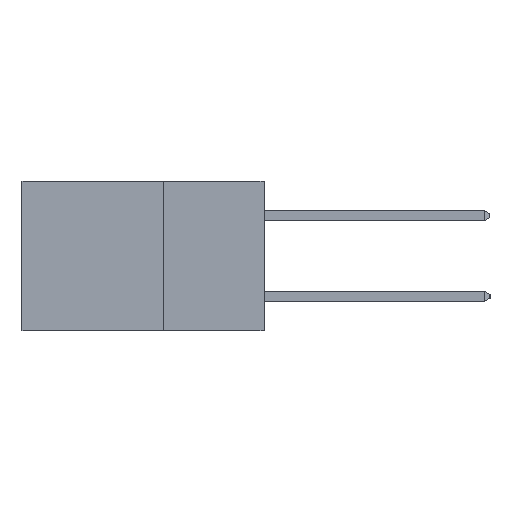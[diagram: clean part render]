
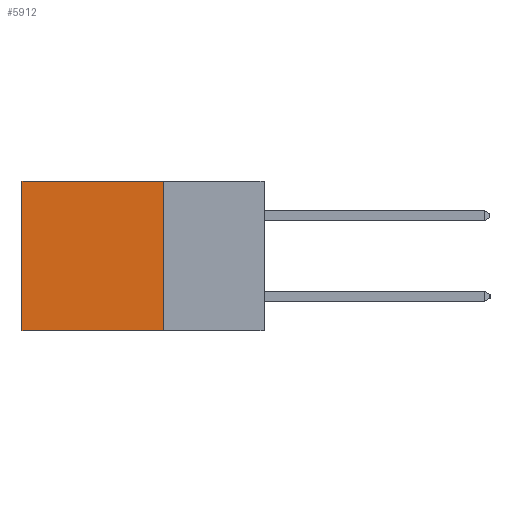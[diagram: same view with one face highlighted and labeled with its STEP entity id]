
A CAD part, left-side view. The second image highlights one B-rep face of the part: STEP entity #5912.
In plain terms, the highlighted planar face has unit normal (-1, 0, 0).
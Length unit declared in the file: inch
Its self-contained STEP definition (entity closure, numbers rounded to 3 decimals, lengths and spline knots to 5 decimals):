
#74 = DIRECTION ( 'NONE',  ( 0., 0., -1. ) ) ;
#512 = CARTESIAN_POINT ( 'NONE',  ( 0.2615, 0.25, -0.37 ) ) ;
#1119 = LINE ( 'NONE', #2760, #7831 ) ;
#1489 = CARTESIAN_POINT ( 'NONE',  ( 0.2615, 0.25, 0. ) ) ;
#1508 = DIRECTION ( 'NONE',  ( 0., 0., -1. ) ) ;
#1572 = LINE ( 'NONE', #512, #10330 ) ;
#2566 = PLANE ( 'NONE',  #3151 ) ;
#2760 = CARTESIAN_POINT ( 'NONE',  ( 0.2615, 0.25, -0.37 ) ) ;
#3151 = AXIS2_PLACEMENT_3D ( 'NONE', #3512, #10119, #5229 ) ;
#3495 = CARTESIAN_POINT ( 'NONE',  ( 0.2615, 0.25, -0.37 ) ) ;
#3512 = CARTESIAN_POINT ( 'NONE',  ( 0.2615, 0.25, -0.37 ) ) ;
#4608 = EDGE_LOOP ( 'NONE', ( #7657, #6684, #6262, #6274 ) ) ;
#4734 = VERTEX_POINT ( 'NONE', #8314 ) ;
#4958 = LINE ( 'NONE', #10411, #9104 ) ;
#4966 = FACE_OUTER_BOUND ( 'NONE', #4608, .T. ) ;
#5229 = DIRECTION ( 'NONE',  ( 0., 0., -1. ) ) ;
#5588 = CARTESIAN_POINT ( 'NONE',  ( 0.2615, 0.6, -0.37 ) ) ;
#5912 = ADVANCED_FACE ( 'NONE', ( #4966 ), #2566, .F. ) ;
#5965 = VERTEX_POINT ( 'NONE', #6165 ) ;
#6045 = EDGE_CURVE ( 'NONE', #6801, #4734, #1119, .T. ) ;
#6165 = CARTESIAN_POINT ( 'NONE',  ( 0.2615, 0.6, 0. ) ) ;
#6214 = EDGE_CURVE ( 'NONE', #5965, #4734, #11045, .T. ) ;
#6262 = ORIENTED_EDGE ( 'NONE', *, *, #7633, .F. ) ;
#6274 = ORIENTED_EDGE ( 'NONE', *, *, #7068, .T. ) ;
#6684 = ORIENTED_EDGE ( 'NONE', *, *, #6045, .F. ) ;
#6801 = VERTEX_POINT ( 'NONE', #3495 ) ;
#7068 = EDGE_CURVE ( 'NONE', #11093, #5965, #4958, .T. ) ;
#7633 = EDGE_CURVE ( 'NONE', #11093, #6801, #1572, .T. ) ;
#7657 = ORIENTED_EDGE ( 'NONE', *, *, #6214, .T. ) ;
#7831 = VECTOR ( 'NONE', #7862, 39.37008 ) ;
#7862 = DIRECTION ( 'NONE',  ( 0., 1., 0. ) ) ;
#8314 = CARTESIAN_POINT ( 'NONE',  ( 0.2615, 0.6, -0.37 ) ) ;
#8712 = VECTOR ( 'NONE', #74, 39.37008 ) ;
#8860 = DIRECTION ( 'NONE',  ( 0., 1., 0. ) ) ;
#9104 = VECTOR ( 'NONE', #8860, 39.37008 ) ;
#10119 = DIRECTION ( 'NONE',  ( 1., 0., 0. ) ) ;
#10330 = VECTOR ( 'NONE', #1508, 39.37008 ) ;
#10411 = CARTESIAN_POINT ( 'NONE',  ( 0.2615, 0.25, 0. ) ) ;
#11045 = LINE ( 'NONE', #5588, #8712 ) ;
#11093 = VERTEX_POINT ( 'NONE', #1489 ) ;
